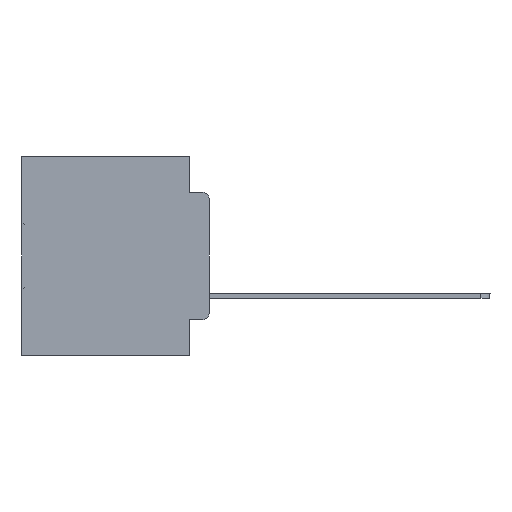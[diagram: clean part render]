
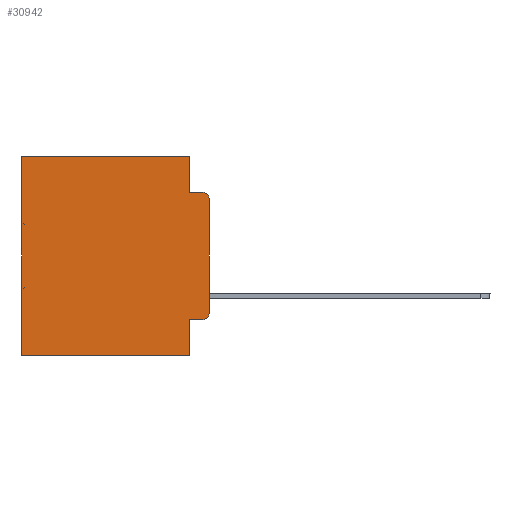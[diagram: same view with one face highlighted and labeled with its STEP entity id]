
A CAD part, left-side view. The second image highlights one B-rep face of the part: STEP entity #30942.
In plain terms, the highlighted planar face has unit normal (-1, 0, 0).
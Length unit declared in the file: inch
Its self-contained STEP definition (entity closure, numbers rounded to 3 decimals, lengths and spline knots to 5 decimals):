
#1540 = VECTOR ( 'NONE', #27753, 39.37008 ) ;
#1849 = VECTOR ( 'NONE', #11086, 39.37008 ) ;
#2135 = ORIENTED_EDGE ( 'NONE', *, *, #30976, .T. ) ;
#2599 = LINE ( 'NONE', #35112, #1849 ) ;
#3015 = LINE ( 'NONE', #33542, #1540 ) ;
#3183 = CARTESIAN_POINT ( 'NONE',  ( 0.298, 0.051, 0. ) ) ;
#4113 = EDGE_CURVE ( 'NONE', #11168, #23004, #11183, .T. ) ;
#4510 = DIRECTION ( 'NONE',  ( 0., 0., -1. ) ) ;
#4647 = DIRECTION ( 'NONE',  ( 0., 0., -1. ) ) ;
#4665 = VECTOR ( 'NONE', #28686, 39.37008 ) ;
#4935 = CARTESIAN_POINT ( 'NONE',  ( 0.298, 0.02, -0.1085 ) ) ;
#5158 = CARTESIAN_POINT ( 'NONE',  ( 0.298, 0.02, -0.4115 ) ) ;
#5607 = EDGE_CURVE ( 'NONE', #21816, #14312, #6666, .T. ) ;
#5689 = CIRCLE ( 'NONE', #14341, 0.02 ) ;
#6625 = LINE ( 'NONE', #15280, #31436 ) ;
#6666 = LINE ( 'NONE', #22558, #4665 ) ;
#7145 = ORIENTED_EDGE ( 'NONE', *, *, #18444, .T. ) ;
#7566 = CIRCLE ( 'NONE', #13348, 0.02 ) ;
#7573 = CARTESIAN_POINT ( 'NONE',  ( 0.298, 0., -0.3915 ) ) ;
#8931 = CARTESIAN_POINT ( 'NONE',  ( 0.298, 0.051, -0.4115 ) ) ;
#9942 = CARTESIAN_POINT ( 'NONE',  ( 0.298, 0.473, 0. ) ) ;
#10210 = EDGE_CURVE ( 'NONE', #11168, #27800, #7566, .T. ) ;
#10537 = DIRECTION ( 'NONE',  ( 0., 0., -1. ) ) ;
#11086 = DIRECTION ( 'NONE',  ( 0., 0., -1. ) ) ;
#11168 = VERTEX_POINT ( 'NONE', #11987 ) ;
#11183 = LINE ( 'NONE', #24549, #12528 ) ;
#11351 = ORIENTED_EDGE ( 'NONE', *, *, #4113, .F. ) ;
#11987 = CARTESIAN_POINT ( 'NONE',  ( 0.298, 0., -0.1085 ) ) ;
#12528 = VECTOR ( 'NONE', #27062, 39.37008 ) ;
#12841 = ORIENTED_EDGE ( 'NONE', *, *, #26239, .F. ) ;
#13348 = AXIS2_PLACEMENT_3D ( 'NONE', #4935, #32401, #10537 ) ;
#13363 = EDGE_LOOP ( 'NONE', ( #11351, #31018, #15809, #27477, #17435, #35005, #20324, #12841, #2135, #7145 ) ) ;
#14312 = VERTEX_POINT ( 'NONE', #28060 ) ;
#14341 = AXIS2_PLACEMENT_3D ( 'NONE', #24338, #18901, #4647 ) ;
#15017 = CARTESIAN_POINT ( 'NONE',  ( 0.298, 0.473, 0. ) ) ;
#15056 = EDGE_CURVE ( 'NONE', #19294, #21590, #3015, .T. ) ;
#15280 = CARTESIAN_POINT ( 'NONE',  ( 0.298, 0.051, -0.0885 ) ) ;
#15809 = ORIENTED_EDGE ( 'NONE', *, *, #30551, .F. ) ;
#16234 = EDGE_CURVE ( 'NONE', #32537, #21590, #29257, .T. ) ;
#17435 = ORIENTED_EDGE ( 'NONE', *, *, #22964, .T. ) ;
#18168 = CARTESIAN_POINT ( 'NONE',  ( 0.298, 0.051, -0.4115 ) ) ;
#18444 = EDGE_CURVE ( 'NONE', #33764, #23004, #5689, .T. ) ;
#18900 = VECTOR ( 'NONE', #4510, 39.37008 ) ;
#18901 = DIRECTION ( 'NONE',  ( -1., 0., 0. ) ) ;
#19294 = VERTEX_POINT ( 'NONE', #26594 ) ;
#19940 = DIRECTION ( 'NONE',  ( 0., 0., -1. ) ) ;
#20324 = ORIENTED_EDGE ( 'NONE', *, *, #15056, .F. ) ;
#20685 = DIRECTION ( 'NONE',  ( 0., -1., 0. ) ) ;
#21590 = VERTEX_POINT ( 'NONE', #24692 ) ;
#21660 = DIRECTION ( 'NONE',  ( 0., 1., 0. ) ) ;
#21816 = VERTEX_POINT ( 'NONE', #3183 ) ;
#22558 = CARTESIAN_POINT ( 'NONE',  ( 0.298, 0.051, 0. ) ) ;
#22657 = LINE ( 'NONE', #8931, #22802 ) ;
#22802 = VECTOR ( 'NONE', #33692, 39.37008 ) ;
#22964 = EDGE_CURVE ( 'NONE', #21816, #32537, #23827, .T. ) ;
#23004 = VERTEX_POINT ( 'NONE', #7573 ) ;
#23216 = CARTESIAN_POINT ( 'NONE',  ( 0.298, 0.02, -0.0885 ) ) ;
#23827 = LINE ( 'NONE', #30152, #31660 ) ;
#24338 = CARTESIAN_POINT ( 'NONE',  ( 0.298, 0.02, -0.3915 ) ) ;
#24549 = CARTESIAN_POINT ( 'NONE',  ( 0.298, 0., 0. ) ) ;
#24692 = CARTESIAN_POINT ( 'NONE',  ( 0.298, 0.473, -0.5 ) ) ;
#24936 = VERTEX_POINT ( 'NONE', #18168 ) ;
#25369 = DIRECTION ( 'NONE',  ( 1., 0., 0. ) ) ;
#26239 = EDGE_CURVE ( 'NONE', #24936, #19294, #2599, .T. ) ;
#26594 = CARTESIAN_POINT ( 'NONE',  ( 0.298, 0.051, -0.5 ) ) ;
#27062 = DIRECTION ( 'NONE',  ( 0., 0., -1. ) ) ;
#27477 = ORIENTED_EDGE ( 'NONE', *, *, #5607, .F. ) ;
#27753 = DIRECTION ( 'NONE',  ( 0., 1., 0. ) ) ;
#27800 = VERTEX_POINT ( 'NONE', #23216 ) ;
#28060 = CARTESIAN_POINT ( 'NONE',  ( 0.298, 0.051, -0.0885 ) ) ;
#28582 = AXIS2_PLACEMENT_3D ( 'NONE', #28974, #25369, #19940 ) ;
#28686 = DIRECTION ( 'NONE',  ( 0., 0., -1. ) ) ;
#28776 = FACE_OUTER_BOUND ( 'NONE', #13363, .T. ) ;
#28974 = CARTESIAN_POINT ( 'NONE',  ( 0.298, 0., 0. ) ) ;
#29257 = LINE ( 'NONE', #9942, #18900 ) ;
#30152 = CARTESIAN_POINT ( 'NONE',  ( 0.298, 0., 0. ) ) ;
#30551 = EDGE_CURVE ( 'NONE', #14312, #27800, #6625, .T. ) ;
#30942 = ADVANCED_FACE ( 'NONE', ( #28776 ), #31146, .F. ) ;
#30976 = EDGE_CURVE ( 'NONE', #24936, #33764, #22657, .T. ) ;
#31018 = ORIENTED_EDGE ( 'NONE', *, *, #10210, .T. ) ;
#31146 = PLANE ( 'NONE',  #28582 ) ;
#31436 = VECTOR ( 'NONE', #20685, 39.37008 ) ;
#31660 = VECTOR ( 'NONE', #21660, 39.37008 ) ;
#32401 = DIRECTION ( 'NONE',  ( -1., 0., 0. ) ) ;
#32537 = VERTEX_POINT ( 'NONE', #15017 ) ;
#33542 = CARTESIAN_POINT ( 'NONE',  ( 0.298, 0., -0.5 ) ) ;
#33692 = DIRECTION ( 'NONE',  ( 0., -1., 0. ) ) ;
#33764 = VERTEX_POINT ( 'NONE', #5158 ) ;
#35005 = ORIENTED_EDGE ( 'NONE', *, *, #16234, .T. ) ;
#35112 = CARTESIAN_POINT ( 'NONE',  ( 0.298, 0.051, 0. ) ) ;
